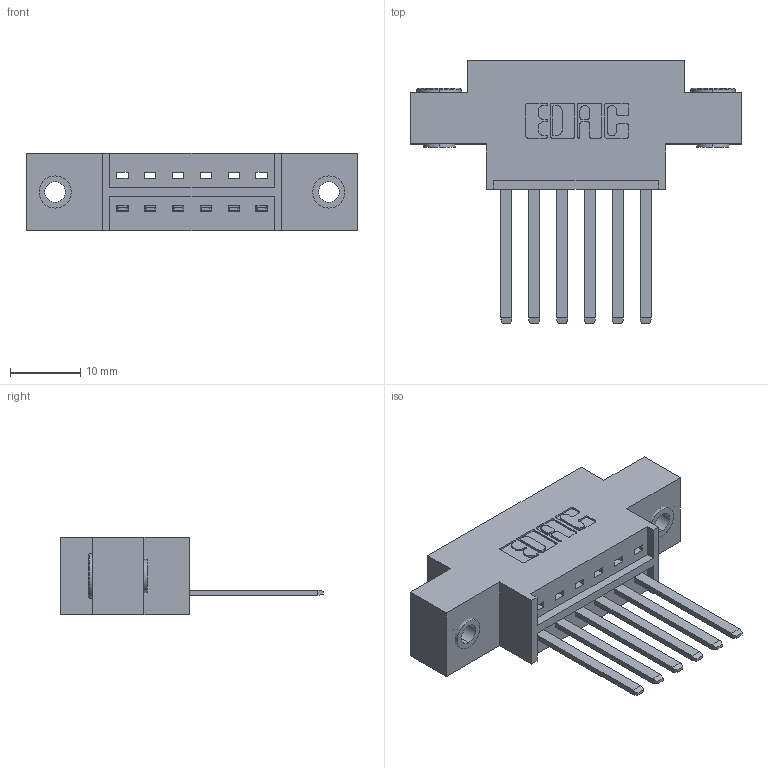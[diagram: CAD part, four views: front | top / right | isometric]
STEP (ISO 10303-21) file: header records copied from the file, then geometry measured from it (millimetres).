
FILE_DESCRIPTION (( 'STEP AP203' ), '1' );
FILE_NAME ('336-006-541-603.STEP', '2020-08-07T19:11:59', ( '' ), ( '' ), 'SwSTEP 2.0', 'SolidWorks 2020', '' );
FILE_SCHEMA (( 'CONFIG_CONTROL_DESIGN' ));
Length unit declared in the file: inch
Products named in the file (4): 336 Part_Offset - .156 Dia - TH; 345-250-002_345-250-002-102; 336-290-001_336-290-541; 336-006-541-603
Assembly tree (9 placements, depth 2):
  336-006-541-603
    336 Part_Offset - .156 Dia - TH
    336-290-001_336-290-541  x6
    345-250-002_345-250-002-102  x2
Bounding box: 47.17 x 37.34 x 11.1 mm (x, y, z)
Volume: 5851 mm3; surface area: 6220.1 mm2
Topology: 9 solids, 9 shells, 456 faces, 1323 edges, 874 vertices
Faces by surface type: plane 288, cylinder 160, cone 8
Entity records: 9617 total; most frequent: CARTESIAN_POINT 1734, ORIENTED_EDGE 1570, DIRECTION 1471, EDGE_CURVE 785, VECTOR 629, LINE 629, VERTEX_POINT 520, AXIS2_PLACEMENT_3D 421
